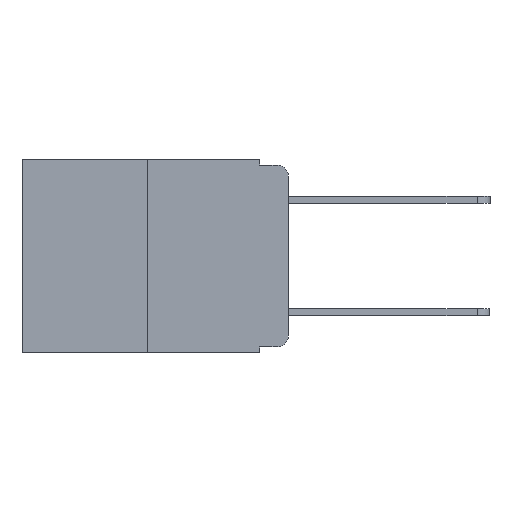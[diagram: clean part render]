
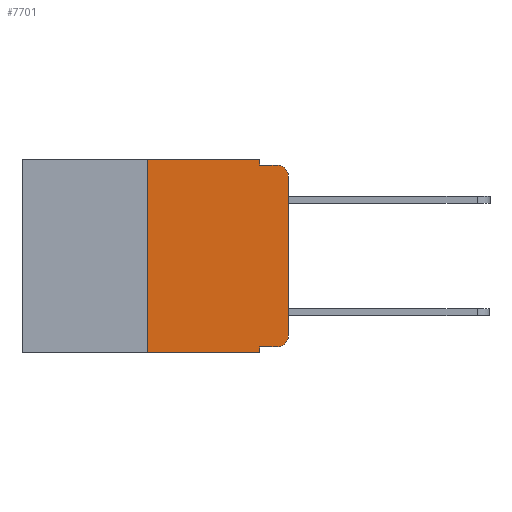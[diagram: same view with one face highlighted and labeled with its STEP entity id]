
A CAD part, left-side view. The second image highlights one B-rep face of the part: STEP entity #7701.
In plain terms, the highlighted planar face has unit normal (-1, 0, 0).
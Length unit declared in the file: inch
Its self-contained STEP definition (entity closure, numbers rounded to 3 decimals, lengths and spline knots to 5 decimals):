
#7 = EDGE_CURVE ( 'NONE', #1727, #1312, #11562, .T. ) ;
#95 = CARTESIAN_POINT ( 'NONE',  ( 0., 0., 0. ) ) ;
#366 = CARTESIAN_POINT ( 'NONE',  ( 0., 0.25, -0.343 ) ) ;
#582 = EDGE_CURVE ( 'NONE', #10208, #9596, #4862, .T. ) ;
#1117 = CARTESIAN_POINT ( 'NONE',  ( 0., 0., -0.03 ) ) ;
#1312 = VERTEX_POINT ( 'NONE', #2787 ) ;
#1576 = CARTESIAN_POINT ( 'NONE',  ( 0., 0.473, 0. ) ) ;
#1674 = DIRECTION ( 'NONE',  ( 0., -1., 0. ) ) ;
#1727 = VERTEX_POINT ( 'NONE', #2339 ) ;
#1867 = EDGE_LOOP ( 'NONE', ( #5588, #11509, #4353, #2477, #4830, #5131, #3371, #9610, #11951, #7667 ) ) ;
#1985 = VECTOR ( 'NONE', #6187, 39.37008 ) ;
#2012 = VERTEX_POINT ( 'NONE', #5199 ) ;
#2054 = VERTEX_POINT ( 'NONE', #5721 ) ;
#2086 = LINE ( 'NONE', #2991, #7622 ) ;
#2286 = EDGE_CURVE ( 'NONE', #8515, #11006, #9310, .T. ) ;
#2305 = LINE ( 'NONE', #6480, #12342 ) ;
#2339 = CARTESIAN_POINT ( 'NONE',  ( 0., 0.051, -0.333 ) ) ;
#2469 = EDGE_CURVE ( 'NONE', #6747, #10208, #2305, .T. ) ;
#2477 = ORIENTED_EDGE ( 'NONE', *, *, #4392, .F. ) ;
#2565 = CARTESIAN_POINT ( 'NONE',  ( 0., 0.051, -0.333 ) ) ;
#2787 = CARTESIAN_POINT ( 'NONE',  ( 0., 0.051, -0.343 ) ) ;
#2882 = LINE ( 'NONE', #8671, #5661 ) ;
#2991 = CARTESIAN_POINT ( 'NONE',  ( 0., 0.473, -0.343 ) ) ;
#3072 = VECTOR ( 'NONE', #3685, 39.37008 ) ;
#3371 = ORIENTED_EDGE ( 'NONE', *, *, #7820, .T. ) ;
#3425 = LINE ( 'NONE', #2565, #3072 ) ;
#3685 = DIRECTION ( 'NONE',  ( 0., -1., 0. ) ) ;
#3852 = PLANE ( 'NONE',  #8700 ) ;
#4353 = ORIENTED_EDGE ( 'NONE', *, *, #4472, .F. ) ;
#4392 = EDGE_CURVE ( 'NONE', #9596, #2012, #2882, .T. ) ;
#4472 = EDGE_CURVE ( 'NONE', #2012, #11006, #7070, .T. ) ;
#4830 = ORIENTED_EDGE ( 'NONE', *, *, #582, .F. ) ;
#4862 = LINE ( 'NONE', #11921, #1985 ) ;
#4886 = DIRECTION ( 'NONE',  ( 1., 0., 0. ) ) ;
#5131 = ORIENTED_EDGE ( 'NONE', *, *, #2469, .F. ) ;
#5199 = CARTESIAN_POINT ( 'NONE',  ( 0., 0.051, -0.01 ) ) ;
#5318 = AXIS2_PLACEMENT_3D ( 'NONE', #10651, #10137, #10114 ) ;
#5390 = DIRECTION ( 'NONE',  ( -1., 0., 0. ) ) ;
#5588 = ORIENTED_EDGE ( 'NONE', *, *, #8059, .T. ) ;
#5661 = VECTOR ( 'NONE', #7737, 39.37008 ) ;
#5721 = CARTESIAN_POINT ( 'NONE',  ( 0., 0., -0.313 ) ) ;
#5882 = CIRCLE ( 'NONE', #6408, 0.02 ) ;
#6187 = DIRECTION ( 'NONE',  ( 0., -1., 0. ) ) ;
#6408 = AXIS2_PLACEMENT_3D ( 'NONE', #11104, #5390, #11989 ) ;
#6433 = CARTESIAN_POINT ( 'NONE',  ( 0., 0.051, 0. ) ) ;
#6480 = CARTESIAN_POINT ( 'NONE',  ( 0., 0.25, 0. ) ) ;
#6542 = LINE ( 'NONE', #95, #9414 ) ;
#6573 = DIRECTION ( 'NONE',  ( 0., 0., 1. ) ) ;
#6595 = DIRECTION ( 'NONE',  ( 0., 0., -1. ) ) ;
#6747 = VERTEX_POINT ( 'NONE', #366 ) ;
#6906 = CARTESIAN_POINT ( 'NONE',  ( 0., 0.051, -0.01 ) ) ;
#7070 = LINE ( 'NONE', #6906, #9348 ) ;
#7082 = DIRECTION ( 'NONE',  ( 0., -1., 0. ) ) ;
#7622 = VECTOR ( 'NONE', #7082, 39.37008 ) ;
#7667 = ORIENTED_EDGE ( 'NONE', *, *, #8498, .T. ) ;
#7701 = ADVANCED_FACE ( 'NONE', ( #8839 ), #3852, .F. ) ;
#7737 = DIRECTION ( 'NONE',  ( 0., 0., -1. ) ) ;
#7820 = EDGE_CURVE ( 'NONE', #6747, #1312, #2086, .T. ) ;
#8021 = CARTESIAN_POINT ( 'NONE',  ( 0., 0.25, 0. ) ) ;
#8059 = EDGE_CURVE ( 'NONE', #2054, #8515, #6542, .T. ) ;
#8492 = DIRECTION ( 'NONE',  ( 0., 0., 1. ) ) ;
#8498 = EDGE_CURVE ( 'NONE', #8931, #2054, #5882, .T. ) ;
#8515 = VERTEX_POINT ( 'NONE', #1117 ) ;
#8671 = CARTESIAN_POINT ( 'NONE',  ( 0., 0.051, 0. ) ) ;
#8700 = AXIS2_PLACEMENT_3D ( 'NONE', #1576, #4886, #11534 ) ;
#8839 = FACE_OUTER_BOUND ( 'NONE', #1867, .T. ) ;
#8931 = VERTEX_POINT ( 'NONE', #11825 ) ;
#9214 = VECTOR ( 'NONE', #6595, 39.37008 ) ;
#9226 = CARTESIAN_POINT ( 'NONE',  ( 0., 0.051, 0. ) ) ;
#9310 = CIRCLE ( 'NONE', #5318, 0.02 ) ;
#9348 = VECTOR ( 'NONE', #1674, 39.37008 ) ;
#9414 = VECTOR ( 'NONE', #8492, 39.37008 ) ;
#9596 = VERTEX_POINT ( 'NONE', #9226 ) ;
#9610 = ORIENTED_EDGE ( 'NONE', *, *, #7, .F. ) ;
#9870 = CARTESIAN_POINT ( 'NONE',  ( 0., 0.02, -0.01 ) ) ;
#10114 = DIRECTION ( 'NONE',  ( 0., 0., -1. ) ) ;
#10137 = DIRECTION ( 'NONE',  ( -1., 0., 0. ) ) ;
#10208 = VERTEX_POINT ( 'NONE', #8021 ) ;
#10651 = CARTESIAN_POINT ( 'NONE',  ( 0., 0.02, -0.03 ) ) ;
#11006 = VERTEX_POINT ( 'NONE', #9870 ) ;
#11104 = CARTESIAN_POINT ( 'NONE',  ( 0., 0.02, -0.313 ) ) ;
#11509 = ORIENTED_EDGE ( 'NONE', *, *, #2286, .T. ) ;
#11534 = DIRECTION ( 'NONE',  ( 0., 0., -1. ) ) ;
#11562 = LINE ( 'NONE', #6433, #9214 ) ;
#11587 = EDGE_CURVE ( 'NONE', #1727, #8931, #3425, .T. ) ;
#11825 = CARTESIAN_POINT ( 'NONE',  ( 0., 0.02, -0.333 ) ) ;
#11921 = CARTESIAN_POINT ( 'NONE',  ( 0., 0.473, 0. ) ) ;
#11951 = ORIENTED_EDGE ( 'NONE', *, *, #11587, .T. ) ;
#11989 = DIRECTION ( 'NONE',  ( 0., 0., -1. ) ) ;
#12342 = VECTOR ( 'NONE', #6573, 39.37008 ) ;
